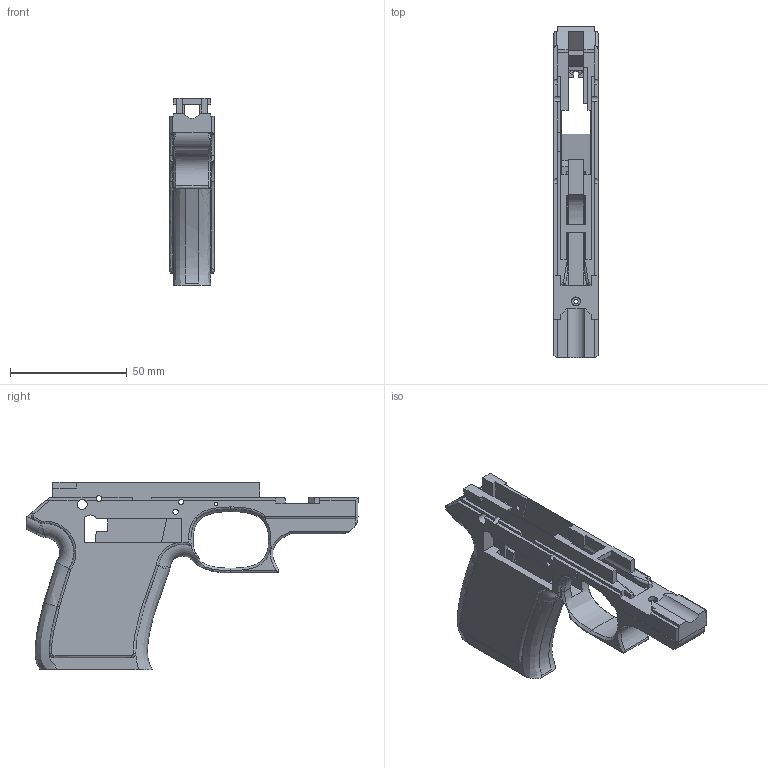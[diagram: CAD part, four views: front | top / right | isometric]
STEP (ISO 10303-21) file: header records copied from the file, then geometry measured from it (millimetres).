
FILE_DESCRIPTION(/* description */ (''),/* implementation_level */ '2;1');
FILE_NAME(/* name */ 'HP22A Receiver v26.step',/* time_stamp */ '2019-12-21T18:24:29-05:00',/* author */ (''),/* organization */ (''),/* preprocessor_version */ 'ST-DEVELOPER v18',/* originating_system */ 'Autodesk Translation Framework v8.12.0.6',/* authorisation */ '');
FILE_SCHEMA (('AUTOMOTIVE_DESIGN { 1 0 10303 214 3 1 1 }'));
Length unit declared in the file: millimetre
Products named in the file (1): HP22A Receiver
Bounding box: 18.9 x 142 x 80 mm (x, y, z)
Volume: 51691.4 mm3; surface area: 28739.3 mm2
Topology: 1 solids, 1 shells, 323 faces, 898 edges, 558 vertices
Faces by surface type: plane 178, bspline 72, cylinder 55, torus 8, sphere 8, cone 2
Full cylindrical faces by diameter (mm): 1.5 x2, 1.8 x1, 2.3 x5, 2.45 x2, 3.85 x2, 4.25 x2, 5 x1
Entity records: 13176 total; most frequent: CARTESIAN_POINT 5292, ORIENTED_EDGE 1792, DIRECTION 1404, EDGE_CURVE 896, LINE 572, VECTOR 572, VERTEX_POINT 558, AXIS2_PLACEMENT_3D 416
